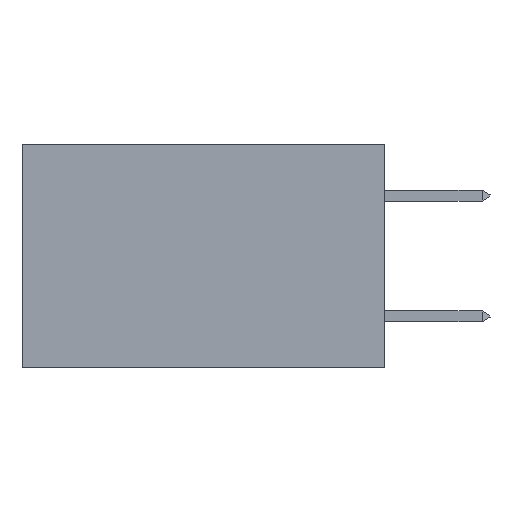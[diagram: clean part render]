
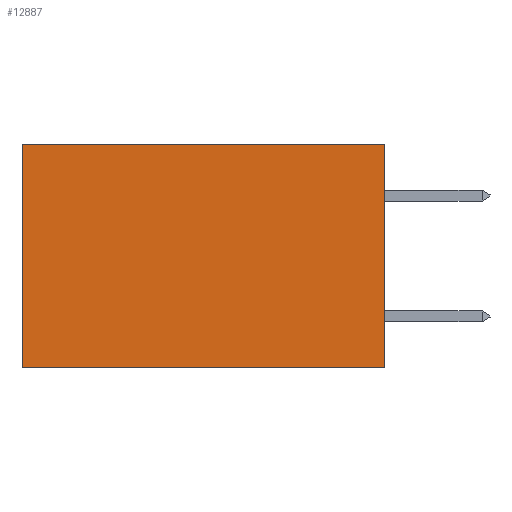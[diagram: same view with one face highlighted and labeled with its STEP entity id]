
A CAD part, left-side view. The second image highlights one B-rep face of the part: STEP entity #12887.
In plain terms, the highlighted planar face has unit normal (-1, 0, 0).
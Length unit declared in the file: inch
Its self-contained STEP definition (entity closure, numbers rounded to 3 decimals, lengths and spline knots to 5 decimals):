
#645 = VERTEX_POINT ( 'NONE', #13185 ) ;
#1318 = CARTESIAN_POINT ( 'NONE',  ( 0.2875, 0., -0.37 ) ) ;
#1677 = DIRECTION ( 'NONE',  ( 0., 0., -1. ) ) ;
#3021 = VECTOR ( 'NONE', #31862, 39.37008 ) ;
#3507 = CARTESIAN_POINT ( 'NONE',  ( 0.2875, 0., 0. ) ) ;
#5428 = EDGE_CURVE ( 'NONE', #645, #17771, #29000, .T. ) ;
#6145 = DIRECTION ( 'NONE',  ( 0., 1., 0. ) ) ;
#7884 = CARTESIAN_POINT ( 'NONE',  ( 0.2875, 0.6, 0. ) ) ;
#12277 = VERTEX_POINT ( 'NONE', #3507 ) ;
#12887 = ADVANCED_FACE ( 'NONE', ( #15171 ), #20778, .F. ) ;
#13185 = CARTESIAN_POINT ( 'NONE',  ( 0.2875, 0., -0.37 ) ) ;
#14059 = LINE ( 'NONE', #25072, #30108 ) ;
#14708 = EDGE_LOOP ( 'NONE', ( #30050, #21407, #31541, #14848 ) ) ;
#14848 = ORIENTED_EDGE ( 'NONE', *, *, #14937, .T. ) ;
#14937 = EDGE_CURVE ( 'NONE', #12277, #15468, #19496, .T. ) ;
#15086 = CARTESIAN_POINT ( 'NONE',  ( 0.2875, 0., 0. ) ) ;
#15171 = FACE_OUTER_BOUND ( 'NONE', #14708, .T. ) ;
#15468 = VERTEX_POINT ( 'NONE', #7884 ) ;
#17091 = AXIS2_PLACEMENT_3D ( 'NONE', #19307, #31449, #20875 ) ;
#17771 = VERTEX_POINT ( 'NONE', #24126 ) ;
#19307 = CARTESIAN_POINT ( 'NONE',  ( 0.2875, 0., 0. ) ) ;
#19496 = LINE ( 'NONE', #15086, #3021 ) ;
#20694 = VECTOR ( 'NONE', #27349, 39.37008 ) ;
#20778 = PLANE ( 'NONE',  #17091 ) ;
#20875 = DIRECTION ( 'NONE',  ( 0., 0., -1. ) ) ;
#21407 = ORIENTED_EDGE ( 'NONE', *, *, #5428, .F. ) ;
#21903 = VECTOR ( 'NONE', #6145, 39.37008 ) ;
#23122 = EDGE_CURVE ( 'NONE', #15468, #17771, #14059, .T. ) ;
#24126 = CARTESIAN_POINT ( 'NONE',  ( 0.2875, 0.6, -0.37 ) ) ;
#24728 = CARTESIAN_POINT ( 'NONE',  ( 0.2875, 0., 0. ) ) ;
#25072 = CARTESIAN_POINT ( 'NONE',  ( 0.2875, 0.6, 0. ) ) ;
#26021 = EDGE_CURVE ( 'NONE', #12277, #645, #33896, .T. ) ;
#27349 = DIRECTION ( 'NONE',  ( 0., 0., -1. ) ) ;
#29000 = LINE ( 'NONE', #1318, #21903 ) ;
#30050 = ORIENTED_EDGE ( 'NONE', *, *, #23122, .T. ) ;
#30108 = VECTOR ( 'NONE', #1677, 39.37008 ) ;
#31449 = DIRECTION ( 'NONE',  ( 1., 0., 0. ) ) ;
#31541 = ORIENTED_EDGE ( 'NONE', *, *, #26021, .F. ) ;
#31862 = DIRECTION ( 'NONE',  ( 0., 1., 0. ) ) ;
#33896 = LINE ( 'NONE', #24728, #20694 ) ;
